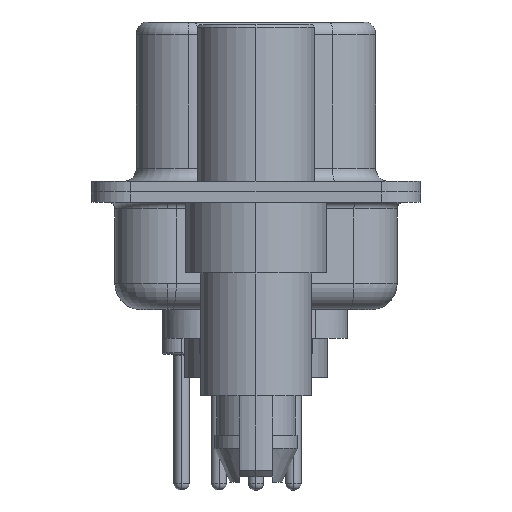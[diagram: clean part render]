
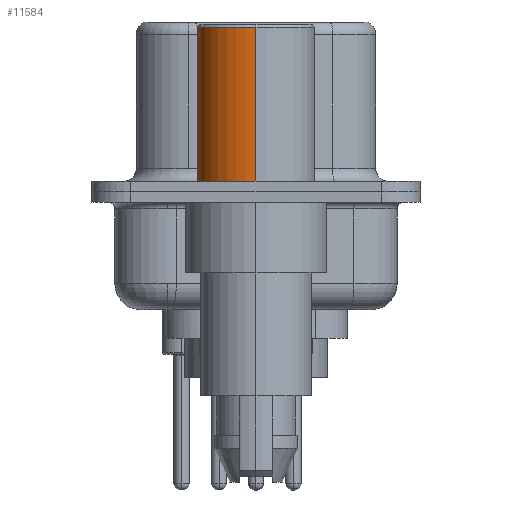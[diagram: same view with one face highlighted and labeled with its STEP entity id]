
A CAD part, left-side view. The second image highlights one B-rep face of the part: STEP entity #11584.
In plain terms, the highlighted cylindrical face has radius 2.25 mm (diameter 4.5 mm), a partial arc.
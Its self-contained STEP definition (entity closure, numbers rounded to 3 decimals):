
#599 = DIRECTION ( 'NONE',  ( 0., 0., 1. ) ) ;
#1750 = CARTESIAN_POINT ( 'NONE',  ( -2.25, 0., 0.4 ) ) ;
#3537 = FACE_OUTER_BOUND ( 'NONE', #23352, .T. ) ;
#4689 = CYLINDRICAL_SURFACE ( 'NONE', #12840, 2.25 ) ;
#4692 = VERTEX_POINT ( 'NONE', #10907 ) ;
#6072 = CARTESIAN_POINT ( 'NONE',  ( -2.25, 0., 6.3 ) ) ;
#6127 = AXIS2_PLACEMENT_3D ( 'NONE', #14123, #17719, #12153 ) ;
#6229 = CARTESIAN_POINT ( 'NONE',  ( 2.25, 0., 0.581 ) ) ;
#8070 = DIRECTION ( 'NONE',  ( 0., 0., 1. ) ) ;
#8228 = EDGE_CURVE ( 'NONE', #20753, #16811, #16195, .T. ) ;
#9062 = CARTESIAN_POINT ( 'NONE',  ( 2.25, 0., 0.4 ) ) ;
#9677 = CARTESIAN_POINT ( 'NONE',  ( 0., 0., 0.581 ) ) ;
#10895 = AXIS2_PLACEMENT_3D ( 'NONE', #16110, #20142, #22012 ) ;
#10907 = CARTESIAN_POINT ( 'NONE',  ( 2.25, 0., 6.3 ) ) ;
#11187 = VECTOR ( 'NONE', #11826, 1000. ) ;
#11584 = ADVANCED_FACE ( 'NONE', ( #3537 ), #4689, .T. ) ;
#11826 = DIRECTION ( 'NONE',  ( 0., 0., 1. ) ) ;
#12153 = DIRECTION ( 'NONE',  ( 1., 0., 0. ) ) ;
#12342 = VECTOR ( 'NONE', #599, 1000. ) ;
#12840 = AXIS2_PLACEMENT_3D ( 'NONE', #9677, #8070, #15257 ) ;
#13364 = ORIENTED_EDGE ( 'NONE', *, *, #18952, .T. ) ;
#14123 = CARTESIAN_POINT ( 'NONE',  ( 0., 0., 6.3 ) ) ;
#14377 = EDGE_CURVE ( 'NONE', #21605, #4692, #14690, .T. ) ;
#14690 = LINE ( 'NONE', #6229, #12342 ) ;
#15257 = DIRECTION ( 'NONE',  ( 1., 0., 0. ) ) ;
#15373 = CARTESIAN_POINT ( 'NONE',  ( -2.25, 0., 0.581 ) ) ;
#15889 = ORIENTED_EDGE ( 'NONE', *, *, #14377, .F. ) ;
#16110 = CARTESIAN_POINT ( 'NONE',  ( 0., 0., 0.4 ) ) ;
#16195 = LINE ( 'NONE', #15373, #11187 ) ;
#16811 = VERTEX_POINT ( 'NONE', #6072 ) ;
#17411 = ORIENTED_EDGE ( 'NONE', *, *, #22040, .F. ) ;
#17719 = DIRECTION ( 'NONE',  ( 0., 0., 1. ) ) ;
#18618 = CIRCLE ( 'NONE', #10895, 2.25 ) ;
#18952 = EDGE_CURVE ( 'NONE', #21605, #20753, #18618, .T. ) ;
#20142 = DIRECTION ( 'NONE',  ( 0., 0., 1. ) ) ;
#20580 = CIRCLE ( 'NONE', #6127, 2.25 ) ;
#20753 = VERTEX_POINT ( 'NONE', #1750 ) ;
#21605 = VERTEX_POINT ( 'NONE', #9062 ) ;
#22012 = DIRECTION ( 'NONE',  ( 1., 0., 0. ) ) ;
#22040 = EDGE_CURVE ( 'NONE', #4692, #16811, #20580, .T. ) ;
#23352 = EDGE_LOOP ( 'NONE', ( #13364, #23849, #17411, #15889 ) ) ;
#23849 = ORIENTED_EDGE ( 'NONE', *, *, #8228, .T. ) ;
